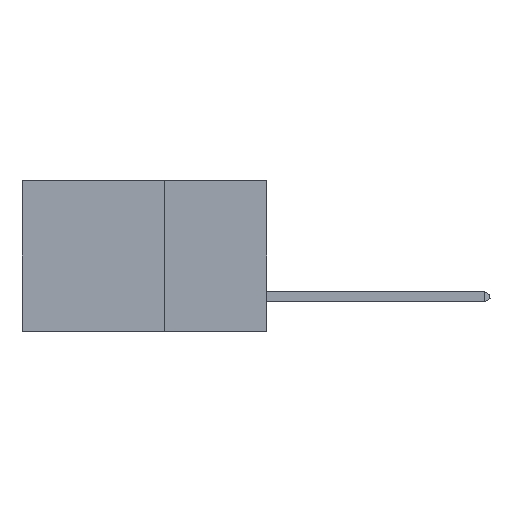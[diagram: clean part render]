
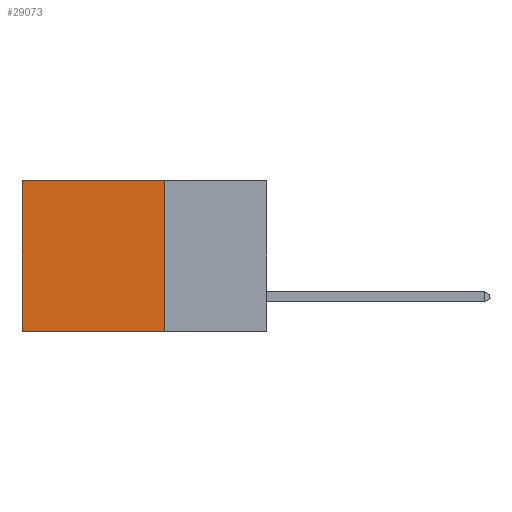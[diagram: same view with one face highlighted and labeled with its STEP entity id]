
A CAD part, left-side view. The second image highlights one B-rep face of the part: STEP entity #29073.
In plain terms, the highlighted planar face has unit normal (-1, 0, 0).
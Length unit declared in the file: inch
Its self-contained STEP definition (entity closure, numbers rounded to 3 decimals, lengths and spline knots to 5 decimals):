
#56 = VERTEX_POINT ( 'NONE', #10037 ) ;
#153 = EDGE_CURVE ( 'NONE', #25902, #9203, #24701, .T. ) ;
#997 = ORIENTED_EDGE ( 'NONE', *, *, #23566, .T. ) ;
#1447 = PLANE ( 'NONE',  #16803 ) ;
#2046 = ORIENTED_EDGE ( 'NONE', *, *, #153, .T. ) ;
#3840 = ORIENTED_EDGE ( 'NONE', *, *, #25119, .F. ) ;
#3856 = CARTESIAN_POINT ( 'NONE',  ( 0.2875, 0.6, 0. ) ) ;
#4010 = EDGE_LOOP ( 'NONE', ( #2046, #23369, #3840, #997 ) ) ;
#4521 = EDGE_CURVE ( 'NONE', #56, #9203, #11769, .T. ) ;
#5486 = DIRECTION ( 'NONE',  ( 1., 0., 0. ) ) ;
#6563 = VECTOR ( 'NONE', #7207, 39.37008 ) ;
#7207 = DIRECTION ( 'NONE',  ( 0., 0., -1. ) ) ;
#8580 = CARTESIAN_POINT ( 'NONE',  ( 0.2875, 0.6, 0. ) ) ;
#9203 = VERTEX_POINT ( 'NONE', #14975 ) ;
#9865 = DIRECTION ( 'NONE',  ( 0., 1., 0. ) ) ;
#10037 = CARTESIAN_POINT ( 'NONE',  ( 0.2875, 0.25, -0.37 ) ) ;
#10085 = CARTESIAN_POINT ( 'NONE',  ( 0.2875, 0.25, 0. ) ) ;
#10119 = VECTOR ( 'NONE', #9865, 39.37008 ) ;
#10469 = FACE_OUTER_BOUND ( 'NONE', #4010, .T. ) ;
#11769 = LINE ( 'NONE', #13973, #23365 ) ;
#12849 = VERTEX_POINT ( 'NONE', #20046 ) ;
#13973 = CARTESIAN_POINT ( 'NONE',  ( 0.2875, 0.25, -0.37 ) ) ;
#14975 = CARTESIAN_POINT ( 'NONE',  ( 0.2875, 0.6, -0.37 ) ) ;
#16803 = AXIS2_PLACEMENT_3D ( 'NONE', #10085, #5486, #18933 ) ;
#18484 = DIRECTION ( 'NONE',  ( 0., 1., 0. ) ) ;
#18933 = DIRECTION ( 'NONE',  ( 0., 0., -1. ) ) ;
#19462 = VECTOR ( 'NONE', #21428, 39.37008 ) ;
#20046 = CARTESIAN_POINT ( 'NONE',  ( 0.2875, 0.25, 0. ) ) ;
#20246 = LINE ( 'NONE', #26930, #6563 ) ;
#21428 = DIRECTION ( 'NONE',  ( 0., 0., -1. ) ) ;
#23319 = CARTESIAN_POINT ( 'NONE',  ( 0.2875, 0.25, 0. ) ) ;
#23365 = VECTOR ( 'NONE', #18484, 39.37008 ) ;
#23369 = ORIENTED_EDGE ( 'NONE', *, *, #4521, .F. ) ;
#23566 = EDGE_CURVE ( 'NONE', #12849, #25902, #26624, .T. ) ;
#24701 = LINE ( 'NONE', #3856, #19462 ) ;
#25119 = EDGE_CURVE ( 'NONE', #12849, #56, #20246, .T. ) ;
#25902 = VERTEX_POINT ( 'NONE', #8580 ) ;
#26624 = LINE ( 'NONE', #23319, #10119 ) ;
#26930 = CARTESIAN_POINT ( 'NONE',  ( 0.2875, 0.25, 0. ) ) ;
#29073 = ADVANCED_FACE ( 'NONE', ( #10469 ), #1447, .F. ) ;
